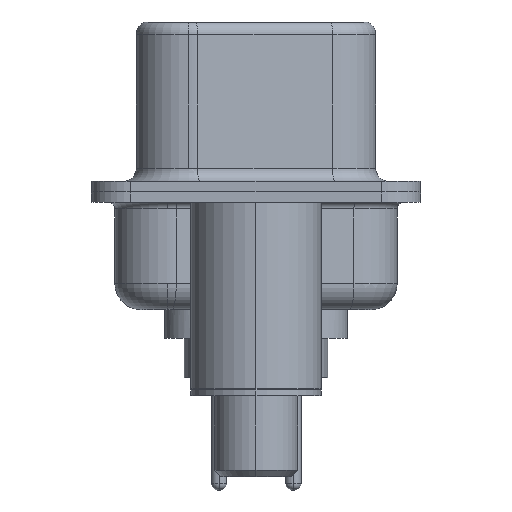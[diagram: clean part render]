
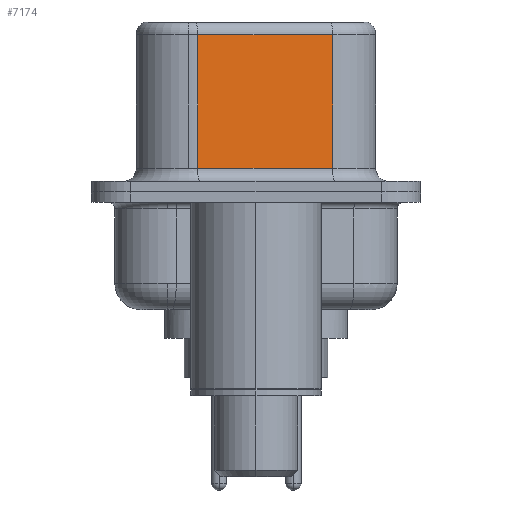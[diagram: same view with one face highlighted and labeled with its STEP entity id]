
A CAD part, left-side view. The second image highlights one B-rep face of the part: STEP entity #7174.
In plain terms, the highlighted planar face has unit normal (-0.985, -0.174, 0).
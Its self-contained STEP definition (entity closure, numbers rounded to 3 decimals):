
#366 = FACE_OUTER_BOUND ( 'NONE', #2012, .T. ) ;
#592 = DIRECTION ( 'NONE',  ( 0., 0., -1. ) ) ;
#664 = EDGE_CURVE ( 'NONE', #783, #5357, #10749, .T. ) ;
#783 = VERTEX_POINT ( 'NONE', #12081 ) ;
#1026 = CARTESIAN_POINT ( 'NONE',  ( 4.565, -2.927, 6.02 ) ) ;
#1162 = DIRECTION ( 'NONE',  ( -0.174, 0.985, 0. ) ) ;
#1236 = DIRECTION ( 'NONE',  ( 0.985, 0.174, 0. ) ) ;
#1296 = VECTOR ( 'NONE', #7568, 1000. ) ;
#1468 = AXIS2_PLACEMENT_3D ( 'NONE', #4240, #1236, #1162 ) ;
#1657 = CARTESIAN_POINT ( 'NONE',  ( 3.655, 2.233, 0.9 ) ) ;
#2012 = EDGE_LOOP ( 'NONE', ( #11101, #15743, #16810, #16444 ) ) ;
#2320 = PLANE ( 'NONE',  #1468 ) ;
#3892 = CARTESIAN_POINT ( 'NONE',  ( 4.565, -2.927, 0.9 ) ) ;
#3971 = CARTESIAN_POINT ( 'NONE',  ( 4.565, -2.927, 6.02 ) ) ;
#4240 = CARTESIAN_POINT ( 'NONE',  ( 4.565, -2.927, 6.52 ) ) ;
#5357 = VERTEX_POINT ( 'NONE', #1657 ) ;
#5504 = DIRECTION ( 'NONE',  ( -0.174, 0.985, 0. ) ) ;
#6553 = VECTOR ( 'NONE', #5504, 1000. ) ;
#7174 = ADVANCED_FACE ( 'NONE', ( #366 ), #2320, .F. ) ;
#7568 = DIRECTION ( 'NONE',  ( 0., 0., -1. ) ) ;
#8409 = EDGE_CURVE ( 'NONE', #17038, #783, #10604, .T. ) ;
#10604 = LINE ( 'NONE', #3971, #6553 ) ;
#10693 = CARTESIAN_POINT ( 'NONE',  ( 4.565, -2.927, 0.9 ) ) ;
#10749 = LINE ( 'NONE', #18216, #18435 ) ;
#11101 = ORIENTED_EDGE ( 'NONE', *, *, #14718, .F. ) ;
#11584 = VECTOR ( 'NONE', #12414, 1000. ) ;
#12081 = CARTESIAN_POINT ( 'NONE',  ( 3.655, 2.233, 6.02 ) ) ;
#12414 = DIRECTION ( 'NONE',  ( 0.174, -0.985, 0. ) ) ;
#13479 = LINE ( 'NONE', #19850, #1296 ) ;
#14718 = EDGE_CURVE ( 'NONE', #17038, #19333, #13479, .T. ) ;
#14833 = EDGE_CURVE ( 'NONE', #5357, #19333, #15634, .T. ) ;
#15634 = LINE ( 'NONE', #10693, #11584 ) ;
#15743 = ORIENTED_EDGE ( 'NONE', *, *, #8409, .T. ) ;
#16444 = ORIENTED_EDGE ( 'NONE', *, *, #14833, .T. ) ;
#16810 = ORIENTED_EDGE ( 'NONE', *, *, #664, .T. ) ;
#17038 = VERTEX_POINT ( 'NONE', #1026 ) ;
#18216 = CARTESIAN_POINT ( 'NONE',  ( 3.655, 2.233, 6.52 ) ) ;
#18435 = VECTOR ( 'NONE', #592, 1000. ) ;
#19333 = VERTEX_POINT ( 'NONE', #3892 ) ;
#19850 = CARTESIAN_POINT ( 'NONE',  ( 4.565, -2.927, 6.52 ) ) ;
